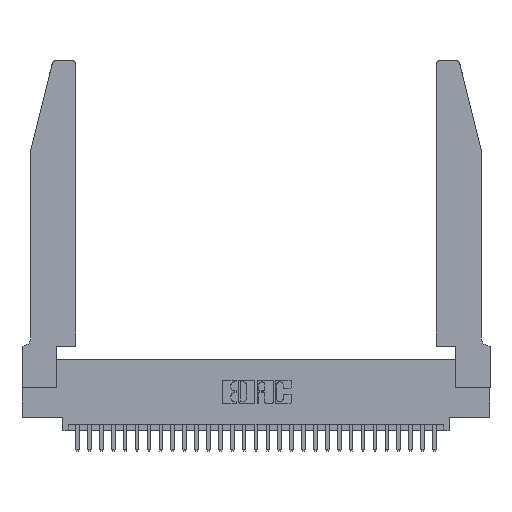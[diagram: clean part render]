
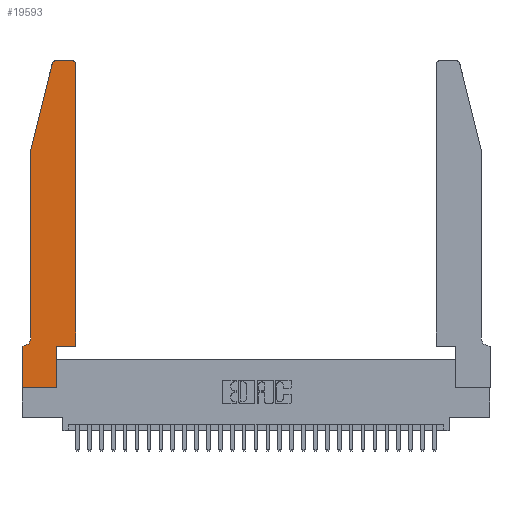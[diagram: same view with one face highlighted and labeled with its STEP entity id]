
A CAD part, top view. The second image highlights one B-rep face of the part: STEP entity #19593.
In plain terms, the highlighted planar face has unit normal (0, 0, 1).
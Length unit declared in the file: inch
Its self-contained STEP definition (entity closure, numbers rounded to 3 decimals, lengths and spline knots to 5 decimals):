
#485 = VECTOR ( 'NONE', #24904, 39.37008 ) ;
#593 = ORIENTED_EDGE ( 'NONE', *, *, #4051, .T. ) ;
#1149 = VERTEX_POINT ( 'NONE', #14331 ) ;
#1170 = ORIENTED_EDGE ( 'NONE', *, *, #8124, .T. ) ;
#1346 = VECTOR ( 'NONE', #2236, 39.37008 ) ;
#1642 = LINE ( 'NONE', #9891, #28086 ) ;
#1746 = ORIENTED_EDGE ( 'NONE', *, *, #28762, .T. ) ;
#2064 = CARTESIAN_POINT ( 'NONE',  ( 0., 0., 0.37 ) ) ;
#2143 = CARTESIAN_POINT ( 'NONE',  ( 0.2605, 2.75, 0.37 ) ) ;
#2236 = DIRECTION ( 'NONE',  ( -1., 0., 0. ) ) ;
#2427 = DIRECTION ( 'NONE',  ( 0., 0., -1. ) ) ;
#2906 = VECTOR ( 'NONE', #21189, 39.37008 ) ;
#3171 = LINE ( 'NONE', #2143, #1346 ) ;
#3444 = VERTEX_POINT ( 'NONE', #4540 ) ;
#3911 = CARTESIAN_POINT ( 'NONE',  ( 0.2865, 0.35, 0.37 ) ) ;
#4051 = EDGE_CURVE ( 'NONE', #18273, #1149, #4879, .T. ) ;
#4540 = CARTESIAN_POINT ( 'NONE',  ( 0.4505, 2.72, 0.37 ) ) ;
#4772 = CARTESIAN_POINT ( 'NONE',  ( 0., 0., 0.37 ) ) ;
#4879 = CIRCLE ( 'NONE', #8419, 0.07 ) ;
#4900 = DIRECTION ( 'NONE',  ( -1., 0., 0. ) ) ;
#5305 = LINE ( 'NONE', #11118, #24758 ) ;
#5530 = CARTESIAN_POINT ( 'NONE',  ( 0.4505, 0.35, 0.37 ) ) ;
#6185 = VERTEX_POINT ( 'NONE', #27580 ) ;
#6679 = ORIENTED_EDGE ( 'NONE', *, *, #30099, .T. ) ;
#6814 = LINE ( 'NONE', #24811, #485 ) ;
#7062 = CARTESIAN_POINT ( 'NONE',  ( 0.284, 2.72, 0.37 ) ) ;
#7179 = DIRECTION ( 'NONE',  ( 0., -1., 0. ) ) ;
#7627 = VERTEX_POINT ( 'NONE', #13463 ) ;
#7885 = EDGE_CURVE ( 'NONE', #6185, #21090, #5305, .T. ) ;
#8124 = EDGE_CURVE ( 'NONE', #16407, #29714, #6814, .T. ) ;
#8419 = AXIS2_PLACEMENT_3D ( 'NONE', #24142, #2427, #4900 ) ;
#9400 = CARTESIAN_POINT ( 'NONE',  ( 0.0755, 2., 0.37 ) ) ;
#9498 = DIRECTION ( 'NONE',  ( 1., 0., 0. ) ) ;
#9875 = CARTESIAN_POINT ( 'NONE',  ( 0.25487, 2.72718, 0.37 ) ) ;
#9891 = CARTESIAN_POINT ( 'NONE',  ( 0.4505, 0.35, 0.37 ) ) ;
#10012 = AXIS2_PLACEMENT_3D ( 'NONE', #18237, #25530, #11675 ) ;
#10506 = DIRECTION ( 'NONE',  ( 0., 0., 1. ) ) ;
#10916 = ORIENTED_EDGE ( 'NONE', *, *, #15304, .T. ) ;
#11033 = CARTESIAN_POINT ( 'NONE',  ( 0.284, 2.75, 0.37 ) ) ;
#11118 = CARTESIAN_POINT ( 'NONE',  ( 0.2865, 0.35, 0.37 ) ) ;
#11222 = VERTEX_POINT ( 'NONE', #30406 ) ;
#11597 = AXIS2_PLACEMENT_3D ( 'NONE', #28718, #10506, #12909 ) ;
#11663 = ORIENTED_EDGE ( 'NONE', *, *, #25092, .T. ) ;
#11675 = DIRECTION ( 'NONE',  ( 1., 0., 0. ) ) ;
#12277 = CIRCLE ( 'NONE', #26953, 0.03 ) ;
#12280 = EDGE_LOOP ( 'NONE', ( #30815, #1746, #1170, #6679, #593, #17230, #24912, #11663, #19981, #17635, #10916, #16954 ) ) ;
#12887 = DIRECTION ( 'NONE',  ( 1., 0., 0. ) ) ;
#12909 = DIRECTION ( 'NONE',  ( 1., 0., 0. ) ) ;
#13463 = CARTESIAN_POINT ( 'NONE',  ( 0.4505, 0.35, 0.37 ) ) ;
#13933 = CARTESIAN_POINT ( 'NONE',  ( 0., 0., 0.37 ) ) ;
#14331 = CARTESIAN_POINT ( 'NONE',  ( 0.0055, 0.35, 0.37 ) ) ;
#15040 = VECTOR ( 'NONE', #26143, 39.37008 ) ;
#15304 = EDGE_CURVE ( 'NONE', #7627, #3444, #1642, .T. ) ;
#15345 = DIRECTION ( 'NONE',  ( 0., -1., 0. ) ) ;
#15644 = PLANE ( 'NONE',  #10012 ) ;
#15926 = CARTESIAN_POINT ( 'NONE',  ( 0., 0.35, 0.37 ) ) ;
#16407 = VERTEX_POINT ( 'NONE', #9875 ) ;
#16954 = ORIENTED_EDGE ( 'NONE', *, *, #27575, .T. ) ;
#17067 = FACE_OUTER_BOUND ( 'NONE', #12280, .T. ) ;
#17230 = ORIENTED_EDGE ( 'NONE', *, *, #22516, .T. ) ;
#17635 = ORIENTED_EDGE ( 'NONE', *, *, #29383, .T. ) ;
#18237 = CARTESIAN_POINT ( 'NONE',  ( 0., 0.35, 0.37 ) ) ;
#18273 = VERTEX_POINT ( 'NONE', #24050 ) ;
#18547 = CARTESIAN_POINT ( 'NONE',  ( 0.0755, 0.35, 0.37 ) ) ;
#18598 = LINE ( 'NONE', #18547, #2906 ) ;
#19583 = VERTEX_POINT ( 'NONE', #11033 ) ;
#19593 = ADVANCED_FACE ( 'NONE', ( #17067 ), #15644, .T. ) ;
#19981 = ORIENTED_EDGE ( 'NONE', *, *, #7885, .T. ) ;
#21090 = VERTEX_POINT ( 'NONE', #3911 ) ;
#21189 = DIRECTION ( 'NONE',  ( -1., 0., 0. ) ) ;
#22042 = EDGE_CURVE ( 'NONE', #27888, #26173, #28297, .T. ) ;
#22516 = EDGE_CURVE ( 'NONE', #1149, #27888, #18598, .T. ) ;
#23067 = LINE ( 'NONE', #24829, #28689 ) ;
#23809 = DIRECTION ( 'NONE',  ( 0., 0., 1. ) ) ;
#23828 = EDGE_CURVE ( 'NONE', #11222, #19583, #3171, .T. ) ;
#23834 = DIRECTION ( 'NONE',  ( 0., 1., 0. ) ) ;
#24050 = CARTESIAN_POINT ( 'NONE',  ( 0.0755, 0.42, 0.37 ) ) ;
#24142 = CARTESIAN_POINT ( 'NONE',  ( 0.0055, 0.42, 0.37 ) ) ;
#24398 = LINE ( 'NONE', #2064, #15040 ) ;
#24499 = DIRECTION ( 'NONE',  ( 0., 1., 0. ) ) ;
#24758 = VECTOR ( 'NONE', #23834, 39.37008 ) ;
#24811 = CARTESIAN_POINT ( 'NONE',  ( 0.0755, 2., 0.37 ) ) ;
#24829 = CARTESIAN_POINT ( 'NONE',  ( 0.0755, 2., 0.37 ) ) ;
#24904 = DIRECTION ( 'NONE',  ( -0.239, -0.971, 0. ) ) ;
#24912 = ORIENTED_EDGE ( 'NONE', *, *, #22042, .T. ) ;
#25092 = EDGE_CURVE ( 'NONE', #26173, #6185, #24398, .T. ) ;
#25530 = DIRECTION ( 'NONE',  ( 0., 0., 1. ) ) ;
#26143 = DIRECTION ( 'NONE',  ( 1., 0., 0. ) ) ;
#26173 = VERTEX_POINT ( 'NONE', #13933 ) ;
#26953 = AXIS2_PLACEMENT_3D ( 'NONE', #7062, #23809, #9498 ) ;
#27161 = VECTOR ( 'NONE', #7179, 39.37008 ) ;
#27508 = LINE ( 'NONE', #5530, #28255 ) ;
#27575 = EDGE_CURVE ( 'NONE', #3444, #11222, #28372, .T. ) ;
#27580 = CARTESIAN_POINT ( 'NONE',  ( 0.2865, 0., 0.37 ) ) ;
#27888 = VERTEX_POINT ( 'NONE', #15926 ) ;
#28086 = VECTOR ( 'NONE', #24499, 39.37008 ) ;
#28255 = VECTOR ( 'NONE', #12887, 39.37008 ) ;
#28297 = LINE ( 'NONE', #4772, #27161 ) ;
#28372 = CIRCLE ( 'NONE', #11597, 0.03 ) ;
#28689 = VECTOR ( 'NONE', #15345, 39.37008 ) ;
#28718 = CARTESIAN_POINT ( 'NONE',  ( 0.4205, 2.72, 0.37 ) ) ;
#28762 = EDGE_CURVE ( 'NONE', #19583, #16407, #12277, .T. ) ;
#29383 = EDGE_CURVE ( 'NONE', #21090, #7627, #27508, .T. ) ;
#29714 = VERTEX_POINT ( 'NONE', #9400 ) ;
#30099 = EDGE_CURVE ( 'NONE', #29714, #18273, #23067, .T. ) ;
#30406 = CARTESIAN_POINT ( 'NONE',  ( 0.4205, 2.75, 0.37 ) ) ;
#30815 = ORIENTED_EDGE ( 'NONE', *, *, #23828, .T. ) ;
